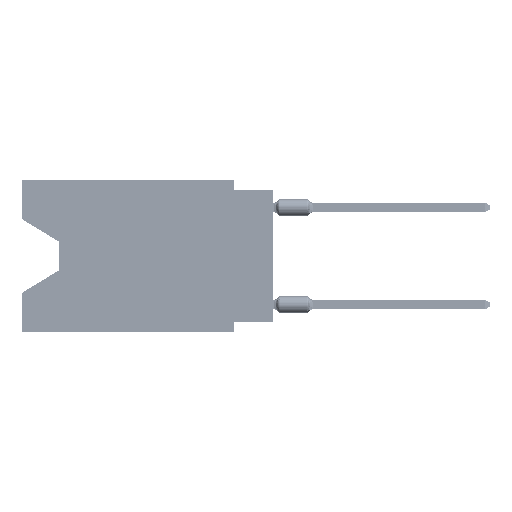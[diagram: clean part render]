
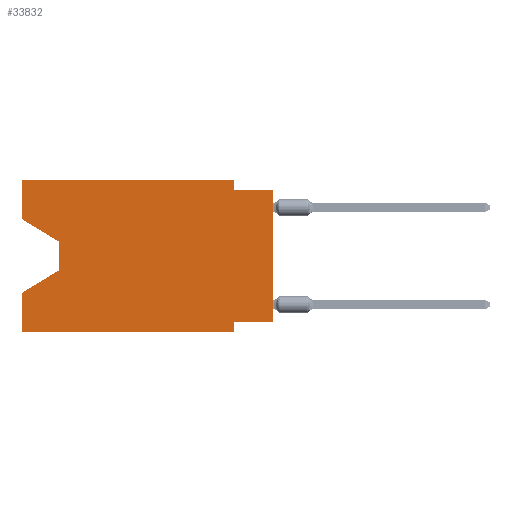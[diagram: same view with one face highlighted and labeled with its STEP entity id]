
A CAD part, left-side view. The second image highlights one B-rep face of the part: STEP entity #33832.
In plain terms, the highlighted planar face has unit normal (-1, 0, 0).
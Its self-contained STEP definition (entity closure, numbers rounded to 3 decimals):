
#657 = VERTEX_POINT ( 'NONE', #72699 ) ;
#3159 = EDGE_CURVE ( 'NONE', #51125, #60322, #71932, .T. ) ;
#3571 = CARTESIAN_POINT ( 'NONE',  ( 0., 16.383, 0. ) ) ;
#3879 = CARTESIAN_POINT ( 'NONE',  ( 0., 2.54, -9.906 ) ) ;
#4636 = DIRECTION ( 'NONE',  ( 0., 0., -1. ) ) ;
#4867 = CARTESIAN_POINT ( 'NONE',  ( 0., 0., 0. ) ) ;
#5792 = VECTOR ( 'NONE', #50566, 1000. ) ;
#6375 = VERTEX_POINT ( 'NONE', #77490 ) ;
#6706 = DIRECTION ( 'NONE',  ( 0., -0.855, -0.519 ) ) ;
#7109 = VERTEX_POINT ( 'NONE', #24206 ) ;
#7381 = DIRECTION ( 'NONE',  ( 0., -1., 0. ) ) ;
#7435 = ORIENTED_EDGE ( 'NONE', *, *, #55383, .T. ) ;
#8219 = VECTOR ( 'NONE', #77142, 1000. ) ;
#8719 = LINE ( 'NONE', #3571, #8984 ) ;
#8984 = VECTOR ( 'NONE', #55694, 1000. ) ;
#12301 = CARTESIAN_POINT ( 'NONE',  ( 0., 16.383, 0. ) ) ;
#12794 = LINE ( 'NONE', #19212, #45535 ) ;
#13227 = CARTESIAN_POINT ( 'NONE',  ( 0., 16.383, -9.906 ) ) ;
#13506 = EDGE_CURVE ( 'NONE', #60584, #63127, #39598, .T. ) ;
#13556 = VECTOR ( 'NONE', #72472, 1000. ) ;
#13749 = CARTESIAN_POINT ( 'NONE',  ( 0., 13.97, -5.893 ) ) ;
#17261 = DIRECTION ( 'NONE',  ( 0., 0., -1. ) ) ;
#17393 = ORIENTED_EDGE ( 'NONE', *, *, #3159, .F. ) ;
#18275 = DIRECTION ( 'NONE',  ( 0., 0., 1. ) ) ;
#19059 = ORIENTED_EDGE ( 'NONE', *, *, #36359, .F. ) ;
#19212 = CARTESIAN_POINT ( 'NONE',  ( 0., 0., -9.271 ) ) ;
#20145 = CARTESIAN_POINT ( 'NONE',  ( 0., 16.383, -2.546 ) ) ;
#22884 = CARTESIAN_POINT ( 'NONE',  ( 0., 16.383, 0. ) ) ;
#23317 = EDGE_CURVE ( 'NONE', #7109, #51125, #66895, .T. ) ;
#23859 = DIRECTION ( 'NONE',  ( 1., 0., 0. ) ) ;
#24206 = CARTESIAN_POINT ( 'NONE',  ( 0., 2.54, 0. ) ) ;
#24273 = LINE ( 'NONE', #76842, #35638 ) ;
#24275 = VECTOR ( 'NONE', #17261, 1000. ) ;
#24576 = VECTOR ( 'NONE', #43813, 1000. ) ;
#26616 = CARTESIAN_POINT ( 'NONE',  ( 0., 0., -0.635 ) ) ;
#27301 = EDGE_CURVE ( 'NONE', #63127, #29779, #74140, .T. ) ;
#29779 = VERTEX_POINT ( 'NONE', #55565 ) ;
#32195 = VERTEX_POINT ( 'NONE', #65045 ) ;
#32542 = VERTEX_POINT ( 'NONE', #13227 ) ;
#33277 = VECTOR ( 'NONE', #81233, 1000. ) ;
#33832 = ADVANCED_FACE ( 'NONE', ( #51189 ), #70870, .F. ) ;
#35638 = VECTOR ( 'NONE', #18275, 1000. ) ;
#36344 = LINE ( 'NONE', #3879, #33277 ) ;
#36359 = EDGE_CURVE ( 'NONE', #6375, #71593, #12794, .T. ) ;
#38498 = VERTEX_POINT ( 'NONE', #72009 ) ;
#39042 = CARTESIAN_POINT ( 'NONE',  ( 0., 13.97, -4.013 ) ) ;
#39180 = CARTESIAN_POINT ( 'NONE',  ( 0., 16.383, -2.546 ) ) ;
#39598 = LINE ( 'NONE', #39180, #75629 ) ;
#40471 = CARTESIAN_POINT ( 'NONE',  ( 0., 2.54, -9.271 ) ) ;
#43813 = DIRECTION ( 'NONE',  ( 0., -1., 0. ) ) ;
#44314 = CARTESIAN_POINT ( 'NONE',  ( 0., 0., -0.635 ) ) ;
#44560 = LINE ( 'NONE', #13749, #61583 ) ;
#45535 = VECTOR ( 'NONE', #79042, 1000. ) ;
#45855 = ORIENTED_EDGE ( 'NONE', *, *, #71466, .F. ) ;
#46200 = EDGE_CURVE ( 'NONE', #6375, #60322, #56559, .T. ) ;
#46695 = ORIENTED_EDGE ( 'NONE', *, *, #27301, .T. ) ;
#50566 = DIRECTION ( 'NONE',  ( 0., 0., 1. ) ) ;
#51125 = VERTEX_POINT ( 'NONE', #75249 ) ;
#51189 = FACE_OUTER_BOUND ( 'NONE', #54809, .T. ) ;
#52180 = ORIENTED_EDGE ( 'NONE', *, *, #80556, .F. ) ;
#54809 = EDGE_LOOP ( 'NONE', ( #76900, #46695, #7435, #52180, #66585, #54863, #19059, #59763, #17393, #75726, #63980, #45855 ) ) ;
#54863 = ORIENTED_EDGE ( 'NONE', *, *, #75994, .F. ) ;
#55383 = EDGE_CURVE ( 'NONE', #29779, #32195, #44560, .T. ) ;
#55565 = CARTESIAN_POINT ( 'NONE',  ( 0., 13.97, -5.893 ) ) ;
#55694 = DIRECTION ( 'NONE',  ( 0., 0., 1. ) ) ;
#55782 = LINE ( 'NONE', #22884, #24576 ) ;
#56559 = LINE ( 'NONE', #4867, #5792 ) ;
#59763 = ORIENTED_EDGE ( 'NONE', *, *, #46200, .T. ) ;
#60322 = VERTEX_POINT ( 'NONE', #44314 ) ;
#60584 = VERTEX_POINT ( 'NONE', #20145 ) ;
#61583 = VECTOR ( 'NONE', #83850, 1000. ) ;
#63127 = VERTEX_POINT ( 'NONE', #39042 ) ;
#63980 = ORIENTED_EDGE ( 'NONE', *, *, #66404, .F. ) ;
#64779 = VECTOR ( 'NONE', #7381, 1000. ) ;
#65045 = CARTESIAN_POINT ( 'NONE',  ( 0., 16.383, -7.36 ) ) ;
#65576 = LINE ( 'NONE', #72420, #8219 ) ;
#66404 = EDGE_CURVE ( 'NONE', #38498, #7109, #55782, .T. ) ;
#66585 = ORIENTED_EDGE ( 'NONE', *, *, #66669, .T. ) ;
#66669 = EDGE_CURVE ( 'NONE', #32542, #657, #65576, .T. ) ;
#66895 = LINE ( 'NONE', #80554, #13556 ) ;
#68563 = CARTESIAN_POINT ( 'NONE',  ( 0., 13.97, -4.013 ) ) ;
#70870 = PLANE ( 'NONE',  #71235 ) ;
#71235 = AXIS2_PLACEMENT_3D ( 'NONE', #12301, #23859, #4636 ) ;
#71466 = EDGE_CURVE ( 'NONE', #60584, #38498, #24273, .T. ) ;
#71593 = VERTEX_POINT ( 'NONE', #40471 ) ;
#71932 = LINE ( 'NONE', #26616, #64779 ) ;
#72009 = CARTESIAN_POINT ( 'NONE',  ( 0., 16.383, 0. ) ) ;
#72420 = CARTESIAN_POINT ( 'NONE',  ( 0., 16.383, -9.906 ) ) ;
#72472 = DIRECTION ( 'NONE',  ( 0., 0., -1. ) ) ;
#72699 = CARTESIAN_POINT ( 'NONE',  ( 0., 2.54, -9.906 ) ) ;
#74140 = LINE ( 'NONE', #68563, #24275 ) ;
#75249 = CARTESIAN_POINT ( 'NONE',  ( 0., 2.54, -0.635 ) ) ;
#75629 = VECTOR ( 'NONE', #6706, 1000. ) ;
#75726 = ORIENTED_EDGE ( 'NONE', *, *, #23317, .F. ) ;
#75994 = EDGE_CURVE ( 'NONE', #71593, #657, #36344, .T. ) ;
#76842 = CARTESIAN_POINT ( 'NONE',  ( 0., 16.383, 0. ) ) ;
#76900 = ORIENTED_EDGE ( 'NONE', *, *, #13506, .T. ) ;
#77142 = DIRECTION ( 'NONE',  ( 0., -1., 0. ) ) ;
#77490 = CARTESIAN_POINT ( 'NONE',  ( 0., 0., -9.271 ) ) ;
#79042 = DIRECTION ( 'NONE',  ( 0., 1., 0. ) ) ;
#80554 = CARTESIAN_POINT ( 'NONE',  ( 0., 2.54, 0. ) ) ;
#80556 = EDGE_CURVE ( 'NONE', #32542, #32195, #8719, .T. ) ;
#81233 = DIRECTION ( 'NONE',  ( 0., 0., -1. ) ) ;
#83850 = DIRECTION ( 'NONE',  ( 0., 0.855, -0.519 ) ) ;
